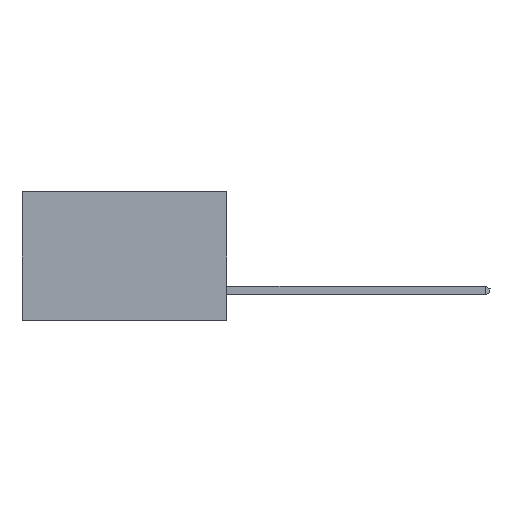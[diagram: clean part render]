
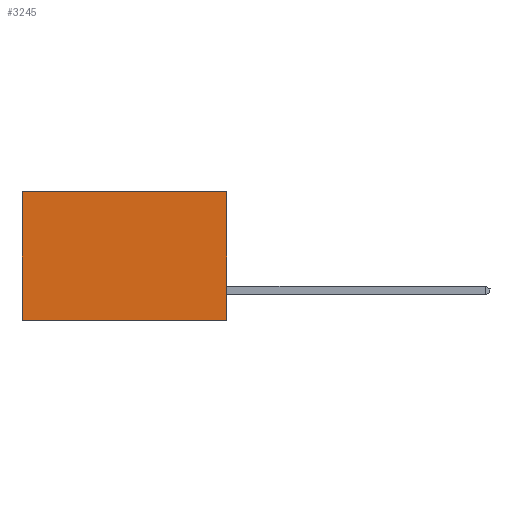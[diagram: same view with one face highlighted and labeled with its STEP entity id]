
A CAD part, left-side view. The second image highlights one B-rep face of the part: STEP entity #3245.
In plain terms, the highlighted planar face has unit normal (-1, 0, 0).
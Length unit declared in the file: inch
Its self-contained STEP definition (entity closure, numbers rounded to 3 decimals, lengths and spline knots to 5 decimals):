
#374 = CARTESIAN_POINT ( 'NONE',  ( 0.277, 0., -0.37 ) ) ;
#1116 = VECTOR ( 'NONE', #10806, 39.37008 ) ;
#1204 = EDGE_CURVE ( 'NONE', #3708, #8304, #6044, .T. ) ;
#1423 = DIRECTION ( 'NONE',  ( 0., 0., -1. ) ) ;
#1908 = ORIENTED_EDGE ( 'NONE', *, *, #4973, .T. ) ;
#1983 = DIRECTION ( 'NONE',  ( 0., 0., -1. ) ) ;
#2627 = EDGE_CURVE ( 'NONE', #3708, #12428, #10683, .T. ) ;
#3245 = ADVANCED_FACE ( 'NONE', ( #4524 ), #7832, .F. ) ;
#3385 = DIRECTION ( 'NONE',  ( 1., 0., 0. ) ) ;
#3577 = AXIS2_PLACEMENT_3D ( 'NONE', #7949, #3385, #1983 ) ;
#3708 = VERTEX_POINT ( 'NONE', #4443 ) ;
#3946 = LINE ( 'NONE', #11336, #1116 ) ;
#4443 = CARTESIAN_POINT ( 'NONE',  ( 0.277, 0., 0. ) ) ;
#4524 = FACE_OUTER_BOUND ( 'NONE', #12166, .T. ) ;
#4973 = EDGE_CURVE ( 'NONE', #8304, #8117, #6808, .T. ) ;
#5493 = CARTESIAN_POINT ( 'NONE',  ( 0.277, 0.59, 0. ) ) ;
#6013 = CARTESIAN_POINT ( 'NONE',  ( 0.277, 0., 0. ) ) ;
#6044 = LINE ( 'NONE', #6013, #8211 ) ;
#6329 = ORIENTED_EDGE ( 'NONE', *, *, #1204, .T. ) ;
#6528 = CARTESIAN_POINT ( 'NONE',  ( 0.277, 0., -0.37 ) ) ;
#6808 = LINE ( 'NONE', #12767, #9657 ) ;
#7559 = EDGE_CURVE ( 'NONE', #12428, #8117, #3946, .T. ) ;
#7825 = ORIENTED_EDGE ( 'NONE', *, *, #7559, .F. ) ;
#7832 = PLANE ( 'NONE',  #3577 ) ;
#7949 = CARTESIAN_POINT ( 'NONE',  ( 0.277, 0., -0.37 ) ) ;
#8117 = VERTEX_POINT ( 'NONE', #10749 ) ;
#8211 = VECTOR ( 'NONE', #10679, 39.37008 ) ;
#8304 = VERTEX_POINT ( 'NONE', #5493 ) ;
#9657 = VECTOR ( 'NONE', #12783, 39.37008 ) ;
#10679 = DIRECTION ( 'NONE',  ( 0., 1., 0. ) ) ;
#10683 = LINE ( 'NONE', #6528, #10995 ) ;
#10749 = CARTESIAN_POINT ( 'NONE',  ( 0.277, 0.59, -0.37 ) ) ;
#10806 = DIRECTION ( 'NONE',  ( 0., 1., 0. ) ) ;
#10995 = VECTOR ( 'NONE', #1423, 39.37008 ) ;
#11273 = ORIENTED_EDGE ( 'NONE', *, *, #2627, .F. ) ;
#11336 = CARTESIAN_POINT ( 'NONE',  ( 0.277, 0., -0.37 ) ) ;
#12166 = EDGE_LOOP ( 'NONE', ( #1908, #7825, #11273, #6329 ) ) ;
#12428 = VERTEX_POINT ( 'NONE', #374 ) ;
#12767 = CARTESIAN_POINT ( 'NONE',  ( 0.277, 0.59, -0.37 ) ) ;
#12783 = DIRECTION ( 'NONE',  ( 0., 0., -1. ) ) ;
